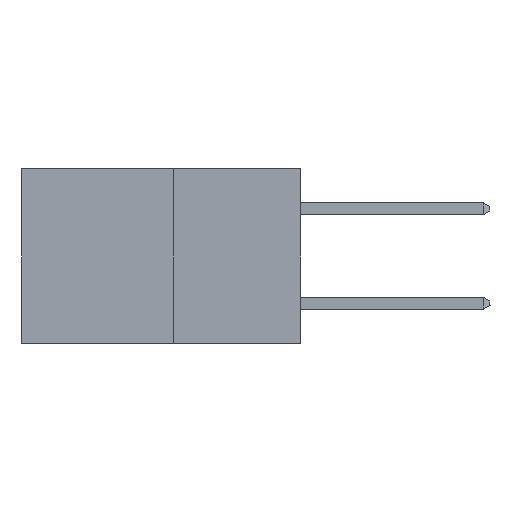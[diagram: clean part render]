
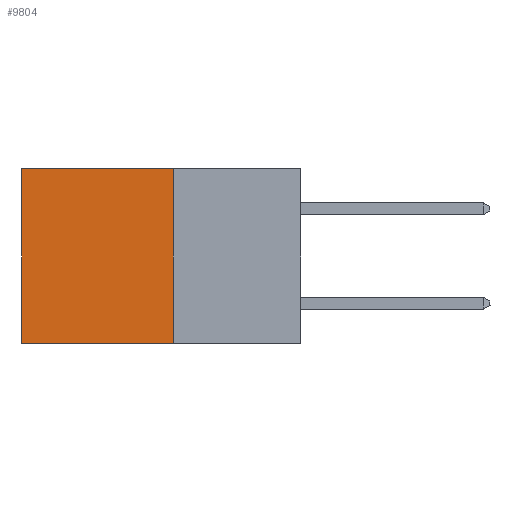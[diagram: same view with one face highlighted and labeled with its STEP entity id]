
A CAD part, left-side view. The second image highlights one B-rep face of the part: STEP entity #9804.
In plain terms, the highlighted planar face has unit normal (-1, 0, 0).
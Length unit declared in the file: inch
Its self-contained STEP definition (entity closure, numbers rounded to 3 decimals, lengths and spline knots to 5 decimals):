
#118 = LINE ( 'NONE', #6475, #18330 ) ;
#1065 = EDGE_CURVE ( 'NONE', #4037, #16688, #16856, .T. ) ;
#1565 = VECTOR ( 'NONE', #26305, 39.37008 ) ;
#2831 = FACE_OUTER_BOUND ( 'NONE', #18908, .T. ) ;
#4037 = VERTEX_POINT ( 'NONE', #20024 ) ;
#6014 = VERTEX_POINT ( 'NONE', #30445 ) ;
#6475 = CARTESIAN_POINT ( 'NONE',  ( 0.277, 0.27, -0.37 ) ) ;
#6865 = DIRECTION ( 'NONE',  ( 0., 0., -1. ) ) ;
#7135 = DIRECTION ( 'NONE',  ( 1., 0., 0. ) ) ;
#7170 = CARTESIAN_POINT ( 'NONE',  ( 0.277, 0.27, -0.37 ) ) ;
#7335 = PLANE ( 'NONE',  #21909 ) ;
#7495 = ORIENTED_EDGE ( 'NONE', *, *, #12129, .T. ) ;
#9587 = DIRECTION ( 'NONE',  ( 0., 1., 0. ) ) ;
#9732 = CARTESIAN_POINT ( 'NONE',  ( 0.277, 0.27, -0.37 ) ) ;
#9804 = ADVANCED_FACE ( 'NONE', ( #2831 ), #7335, .F. ) ;
#10516 = VECTOR ( 'NONE', #18213, 39.37008 ) ;
#10629 = CARTESIAN_POINT ( 'NONE',  ( 0.277, 0.27, 0. ) ) ;
#11913 = EDGE_CURVE ( 'NONE', #6014, #16688, #118, .T. ) ;
#12129 = EDGE_CURVE ( 'NONE', #19293, #4037, #17569, .T. ) ;
#13420 = EDGE_CURVE ( 'NONE', #19293, #6014, #18988, .T. ) ;
#13987 = ORIENTED_EDGE ( 'NONE', *, *, #11913, .F. ) ;
#14429 = CARTESIAN_POINT ( 'NONE',  ( 0.277, 0.59, -0.37 ) ) ;
#16688 = VERTEX_POINT ( 'NONE', #20606 ) ;
#16856 = LINE ( 'NONE', #14429, #10516 ) ;
#17569 = LINE ( 'NONE', #28512, #28590 ) ;
#18213 = DIRECTION ( 'NONE',  ( 0., 0., -1. ) ) ;
#18330 = VECTOR ( 'NONE', #20745, 39.37008 ) ;
#18849 = ORIENTED_EDGE ( 'NONE', *, *, #13420, .F. ) ;
#18908 = EDGE_LOOP ( 'NONE', ( #19523, #13987, #18849, #7495 ) ) ;
#18988 = LINE ( 'NONE', #9732, #1565 ) ;
#19293 = VERTEX_POINT ( 'NONE', #10629 ) ;
#19523 = ORIENTED_EDGE ( 'NONE', *, *, #1065, .T. ) ;
#20024 = CARTESIAN_POINT ( 'NONE',  ( 0.277, 0.59, 0. ) ) ;
#20606 = CARTESIAN_POINT ( 'NONE',  ( 0.277, 0.59, -0.37 ) ) ;
#20745 = DIRECTION ( 'NONE',  ( 0., 1., 0. ) ) ;
#21909 = AXIS2_PLACEMENT_3D ( 'NONE', #7170, #7135, #6865 ) ;
#26305 = DIRECTION ( 'NONE',  ( 0., 0., -1. ) ) ;
#28512 = CARTESIAN_POINT ( 'NONE',  ( 0.277, 0.27, 0. ) ) ;
#28590 = VECTOR ( 'NONE', #9587, 39.37008 ) ;
#30445 = CARTESIAN_POINT ( 'NONE',  ( 0.277, 0.27, -0.37 ) ) ;
